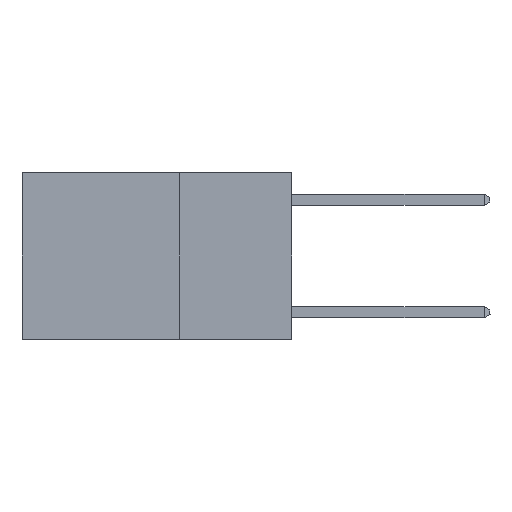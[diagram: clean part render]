
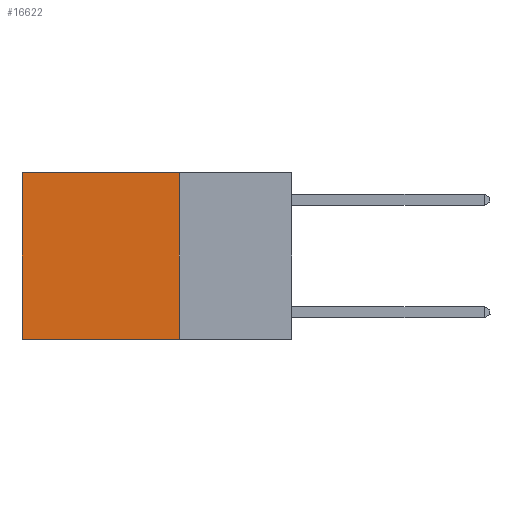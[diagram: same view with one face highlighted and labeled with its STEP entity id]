
A CAD part, left-side view. The second image highlights one B-rep face of the part: STEP entity #16622.
In plain terms, the highlighted planar face has unit normal (-1, 0, 0).
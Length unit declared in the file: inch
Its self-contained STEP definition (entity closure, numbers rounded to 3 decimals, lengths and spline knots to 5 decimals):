
#1301 = VECTOR ( 'NONE', #5866, 39.37008 ) ;
#1638 = DIRECTION ( 'NONE',  ( 0., 1., 0. ) ) ;
#1866 = LINE ( 'NONE', #13395, #1301 ) ;
#3289 = DIRECTION ( 'NONE',  ( 0., 1., 0. ) ) ;
#3380 = FACE_OUTER_BOUND ( 'NONE', #4596, .T. ) ;
#3473 = LINE ( 'NONE', #16441, #8398 ) ;
#3763 = ORIENTED_EDGE ( 'NONE', *, *, #4538, .F. ) ;
#4164 = CARTESIAN_POINT ( 'NONE',  ( 0.2625, 0.25, 0. ) ) ;
#4538 = EDGE_CURVE ( 'NONE', #10761, #7792, #1866, .T. ) ;
#4596 = EDGE_LOOP ( 'NONE', ( #10993, #5463, #3763, #4623 ) ) ;
#4623 = ORIENTED_EDGE ( 'NONE', *, *, #7901, .T. ) ;
#5463 = ORIENTED_EDGE ( 'NONE', *, *, #23384, .F. ) ;
#5664 = EDGE_CURVE ( 'NONE', #13085, #18773, #20598, .T. ) ;
#5866 = DIRECTION ( 'NONE',  ( 0., 0., -1. ) ) ;
#7792 = VERTEX_POINT ( 'NONE', #16129 ) ;
#7901 = EDGE_CURVE ( 'NONE', #10761, #13085, #3473, .T. ) ;
#8398 = VECTOR ( 'NONE', #1638, 39.37008 ) ;
#9588 = VECTOR ( 'NONE', #3289, 39.37008 ) ;
#10697 = CARTESIAN_POINT ( 'NONE',  ( 0.2625, 0.6, 0. ) ) ;
#10749 = LINE ( 'NONE', #12625, #9588 ) ;
#10761 = VERTEX_POINT ( 'NONE', #4164 ) ;
#10781 = VECTOR ( 'NONE', #12615, 39.37008 ) ;
#10993 = ORIENTED_EDGE ( 'NONE', *, *, #5664, .T. ) ;
#11863 = CARTESIAN_POINT ( 'NONE',  ( 0.2625, 0.6, -0.37 ) ) ;
#12300 = DIRECTION ( 'NONE',  ( 0., 0., -1. ) ) ;
#12615 = DIRECTION ( 'NONE',  ( 0., 0., -1. ) ) ;
#12625 = CARTESIAN_POINT ( 'NONE',  ( 0.2625, 0.25, -0.37 ) ) ;
#12809 = AXIS2_PLACEMENT_3D ( 'NONE', #15924, #23284, #12300 ) ;
#13085 = VERTEX_POINT ( 'NONE', #14028 ) ;
#13395 = CARTESIAN_POINT ( 'NONE',  ( 0.2625, 0.25, 0. ) ) ;
#14028 = CARTESIAN_POINT ( 'NONE',  ( 0.2625, 0.6, 0. ) ) ;
#15924 = CARTESIAN_POINT ( 'NONE',  ( 0.2625, 0.25, 0. ) ) ;
#16129 = CARTESIAN_POINT ( 'NONE',  ( 0.2625, 0.25, -0.37 ) ) ;
#16441 = CARTESIAN_POINT ( 'NONE',  ( 0.2625, 0.25, 0. ) ) ;
#16622 = ADVANCED_FACE ( 'NONE', ( #3380 ), #21464, .F. ) ;
#18773 = VERTEX_POINT ( 'NONE', #11863 ) ;
#20598 = LINE ( 'NONE', #10697, #10781 ) ;
#21464 = PLANE ( 'NONE',  #12809 ) ;
#23284 = DIRECTION ( 'NONE',  ( 1., 0., 0. ) ) ;
#23384 = EDGE_CURVE ( 'NONE', #7792, #18773, #10749, .T. ) ;
